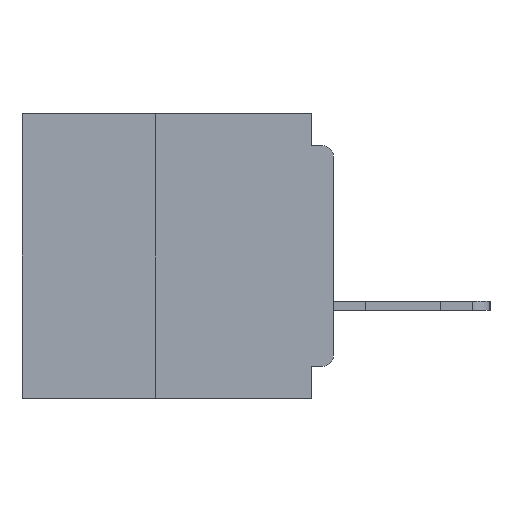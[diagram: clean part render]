
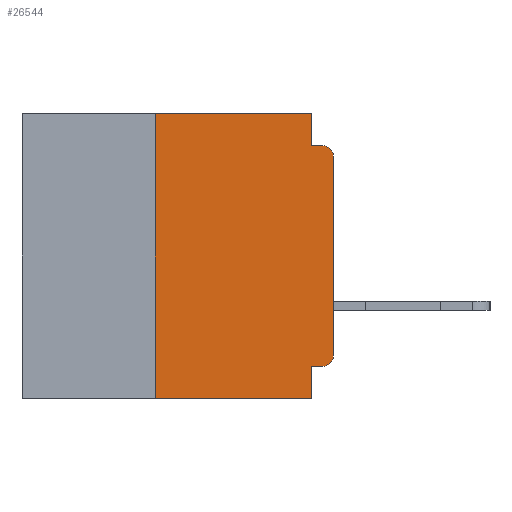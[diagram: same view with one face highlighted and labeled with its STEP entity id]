
A CAD part, left-side view. The second image highlights one B-rep face of the part: STEP entity #26544.
In plain terms, the highlighted planar face has unit normal (-1, 0, 0).
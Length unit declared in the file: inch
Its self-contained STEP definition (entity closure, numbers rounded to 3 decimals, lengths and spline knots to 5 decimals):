
#325 = CARTESIAN_POINT ( 'NONE',  ( 0., 0.015, -0.355 ) ) ;
#611 = DIRECTION ( 'NONE',  ( -1., 0., 0. ) ) ;
#1009 = ORIENTED_EDGE ( 'NONE', *, *, #4591, .T. ) ;
#2400 = VECTOR ( 'NONE', #35543, 39.37008 ) ;
#2461 = CIRCLE ( 'NONE', #37340, 0.015 ) ;
#2537 = ORIENTED_EDGE ( 'NONE', *, *, #14559, .F. ) ;
#3294 = DIRECTION ( 'NONE',  ( 0., -1., 0. ) ) ;
#3856 = LINE ( 'NONE', #5243, #15206 ) ;
#3870 = EDGE_CURVE ( 'NONE', #24639, #48165, #24454, .T. ) ;
#4591 = EDGE_CURVE ( 'NONE', #48165, #49123, #40938, .T. ) ;
#4621 = CARTESIAN_POINT ( 'NONE',  ( 0., 0.031, 0. ) ) ;
#5243 = CARTESIAN_POINT ( 'NONE',  ( 0., 0.031, -0.4 ) ) ;
#5523 = CARTESIAN_POINT ( 'NONE',  ( 0., 0.437, 0. ) ) ;
#5814 = CARTESIAN_POINT ( 'NONE',  ( 0., 0.031, -0.355 ) ) ;
#7251 = ORIENTED_EDGE ( 'NONE', *, *, #16130, .T. ) ;
#7894 = ORIENTED_EDGE ( 'NONE', *, *, #38380, .F. ) ;
#8494 = LINE ( 'NONE', #36701, #29759 ) ;
#8605 = EDGE_CURVE ( 'NONE', #29137, #36766, #36311, .T. ) ;
#9026 = LINE ( 'NONE', #26119, #19013 ) ;
#9439 = PLANE ( 'NONE',  #13709 ) ;
#11237 = ORIENTED_EDGE ( 'NONE', *, *, #13742, .F. ) ;
#11388 = CARTESIAN_POINT ( 'NONE',  ( 0., 0., -0.045 ) ) ;
#11715 = DIRECTION ( 'NONE',  ( 0., 0., -1. ) ) ;
#12145 = CARTESIAN_POINT ( 'NONE',  ( 0., 0.031, -0.4 ) ) ;
#12686 = CARTESIAN_POINT ( 'NONE',  ( 0., 0.25, -0.4 ) ) ;
#13709 = AXIS2_PLACEMENT_3D ( 'NONE', #5523, #39538, #14099 ) ;
#13742 = EDGE_CURVE ( 'NONE', #36766, #52946, #3856, .T. ) ;
#13927 = LINE ( 'NONE', #49802, #23938 ) ;
#14086 = EDGE_CURVE ( 'NONE', #51889, #37253, #13927, .T. ) ;
#14099 = DIRECTION ( 'NONE',  ( 0., 0., -1. ) ) ;
#14559 = EDGE_CURVE ( 'NONE', #37253, #49123, #32463, .T. ) ;
#15206 = VECTOR ( 'NONE', #26446, 39.37008 ) ;
#15401 = LINE ( 'NONE', #15964, #37963 ) ;
#15964 = CARTESIAN_POINT ( 'NONE',  ( 0., 0.437, 0. ) ) ;
#16130 = EDGE_CURVE ( 'NONE', #19442, #52946, #9026, .T. ) ;
#16776 = DIRECTION ( 'NONE',  ( 0., 0., 1. ) ) ;
#16959 = CARTESIAN_POINT ( 'NONE',  ( 0., 0., 0. ) ) ;
#18623 = EDGE_CURVE ( 'NONE', #22688, #51889, #15401, .T. ) ;
#19013 = VECTOR ( 'NONE', #43182, 39.37008 ) ;
#19442 = VERTEX_POINT ( 'NONE', #12686 ) ;
#20889 = CARTESIAN_POINT ( 'NONE',  ( 0., 0.015, -0.045 ) ) ;
#21179 = EDGE_LOOP ( 'NONE', ( #24311, #1009, #2537, #36462, #40455, #7894, #7251, #11237, #45173, #49146 ) ) ;
#21245 = DIRECTION ( 'NONE',  ( 0., 0., -1. ) ) ;
#21297 = DIRECTION ( 'NONE',  ( -1., 0., 0. ) ) ;
#21497 = CARTESIAN_POINT ( 'NONE',  ( 0., 0.015, -0.06 ) ) ;
#22688 = VERTEX_POINT ( 'NONE', #45413 ) ;
#23144 = VECTOR ( 'NONE', #16776, 39.37008 ) ;
#23938 = VECTOR ( 'NONE', #11715, 39.37008 ) ;
#24311 = ORIENTED_EDGE ( 'NONE', *, *, #3870, .T. ) ;
#24454 = LINE ( 'NONE', #16959, #23144 ) ;
#24490 = AXIS2_PLACEMENT_3D ( 'NONE', #21497, #21297, #21245 ) ;
#24639 = VERTEX_POINT ( 'NONE', #41636 ) ;
#26095 = CARTESIAN_POINT ( 'NONE',  ( 0., 0.015, -0.34 ) ) ;
#26119 = CARTESIAN_POINT ( 'NONE',  ( 0., 0.437, -0.4 ) ) ;
#26446 = DIRECTION ( 'NONE',  ( 0., 0., -1. ) ) ;
#26544 = ADVANCED_FACE ( 'NONE', ( #37839 ), #9439, .F. ) ;
#29137 = VERTEX_POINT ( 'NONE', #325 ) ;
#29759 = VECTOR ( 'NONE', #40962, 39.37008 ) ;
#30336 = DIRECTION ( 'NONE',  ( 0., 0., -1. ) ) ;
#31258 = CARTESIAN_POINT ( 'NONE',  ( 0., 0., -0.355 ) ) ;
#32463 = LINE ( 'NONE', #11388, #43767 ) ;
#35543 = DIRECTION ( 'NONE',  ( 0., 1., 0. ) ) ;
#36311 = LINE ( 'NONE', #31258, #2400 ) ;
#36462 = ORIENTED_EDGE ( 'NONE', *, *, #14086, .F. ) ;
#36701 = CARTESIAN_POINT ( 'NONE',  ( 0., 0.25, -0.4 ) ) ;
#36766 = VERTEX_POINT ( 'NONE', #5814 ) ;
#37253 = VERTEX_POINT ( 'NONE', #45189 ) ;
#37340 = AXIS2_PLACEMENT_3D ( 'NONE', #26095, #611, #30336 ) ;
#37369 = CARTESIAN_POINT ( 'NONE',  ( 0., 0., -0.06 ) ) ;
#37839 = FACE_OUTER_BOUND ( 'NONE', #21179, .T. ) ;
#37963 = VECTOR ( 'NONE', #3294, 39.37008 ) ;
#38380 = EDGE_CURVE ( 'NONE', #19442, #22688, #8494, .T. ) ;
#38725 = EDGE_CURVE ( 'NONE', #29137, #24639, #2461, .T. ) ;
#39538 = DIRECTION ( 'NONE',  ( 1., 0., 0. ) ) ;
#40455 = ORIENTED_EDGE ( 'NONE', *, *, #18623, .F. ) ;
#40938 = CIRCLE ( 'NONE', #24490, 0.015 ) ;
#40962 = DIRECTION ( 'NONE',  ( 0., 0., 1. ) ) ;
#41116 = DIRECTION ( 'NONE',  ( 0., -1., 0. ) ) ;
#41636 = CARTESIAN_POINT ( 'NONE',  ( 0., 0., -0.34 ) ) ;
#43182 = DIRECTION ( 'NONE',  ( 0., -1., 0. ) ) ;
#43767 = VECTOR ( 'NONE', #41116, 39.37008 ) ;
#45173 = ORIENTED_EDGE ( 'NONE', *, *, #8605, .F. ) ;
#45189 = CARTESIAN_POINT ( 'NONE',  ( 0., 0.031, -0.045 ) ) ;
#45413 = CARTESIAN_POINT ( 'NONE',  ( 0., 0.25, 0. ) ) ;
#48165 = VERTEX_POINT ( 'NONE', #37369 ) ;
#49123 = VERTEX_POINT ( 'NONE', #20889 ) ;
#49146 = ORIENTED_EDGE ( 'NONE', *, *, #38725, .T. ) ;
#49802 = CARTESIAN_POINT ( 'NONE',  ( 0., 0.031, 0. ) ) ;
#51889 = VERTEX_POINT ( 'NONE', #4621 ) ;
#52946 = VERTEX_POINT ( 'NONE', #12145 ) ;
